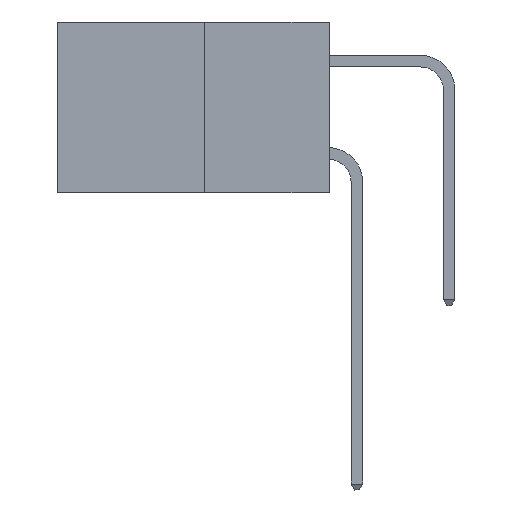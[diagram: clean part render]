
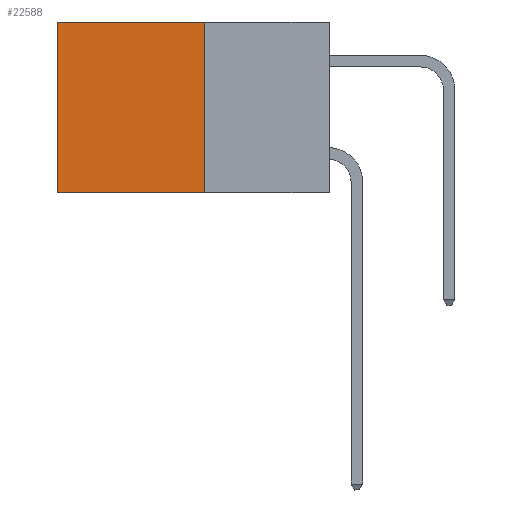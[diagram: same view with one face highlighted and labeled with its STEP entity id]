
A CAD part, left-side view. The second image highlights one B-rep face of the part: STEP entity #22588.
In plain terms, the highlighted planar face has unit normal (-1, 0, 0).
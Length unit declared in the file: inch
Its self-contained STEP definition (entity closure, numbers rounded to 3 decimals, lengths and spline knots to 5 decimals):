
#308 = CARTESIAN_POINT ( 'NONE',  ( 0.277, 0.59, -0.37 ) ) ;
#2342 = LINE ( 'NONE', #20763, #28300 ) ;
#3010 = EDGE_CURVE ( 'NONE', #12105, #6111, #3802, .T. ) ;
#3478 = VECTOR ( 'NONE', #12565, 39.37008 ) ;
#3586 = EDGE_CURVE ( 'NONE', #12547, #6111, #19298, .T. ) ;
#3802 = LINE ( 'NONE', #15116, #10054 ) ;
#4331 = ORIENTED_EDGE ( 'NONE', *, *, #3586, .T. ) ;
#5370 = CARTESIAN_POINT ( 'NONE',  ( 0.277, 0.59, -0.37 ) ) ;
#6111 = VERTEX_POINT ( 'NONE', #5370 ) ;
#6252 = ORIENTED_EDGE ( 'NONE', *, *, #20734, .T. ) ;
#8834 = ORIENTED_EDGE ( 'NONE', *, *, #14954, .F. ) ;
#9442 = DIRECTION ( 'NONE',  ( 1., 0., 0. ) ) ;
#9669 = CARTESIAN_POINT ( 'NONE',  ( 0.277, 0.27, -0.37 ) ) ;
#9868 = CARTESIAN_POINT ( 'NONE',  ( 0.277, 0.27, -0.37 ) ) ;
#10054 = VECTOR ( 'NONE', #14972, 39.37008 ) ;
#11370 = LINE ( 'NONE', #9868, #3478 ) ;
#11796 = FACE_OUTER_BOUND ( 'NONE', #18900, .T. ) ;
#12105 = VERTEX_POINT ( 'NONE', #9669 ) ;
#12182 = AXIS2_PLACEMENT_3D ( 'NONE', #24918, #9442, #27447 ) ;
#12547 = VERTEX_POINT ( 'NONE', #26880 ) ;
#12565 = DIRECTION ( 'NONE',  ( 0., 0., -1. ) ) ;
#12875 = VERTEX_POINT ( 'NONE', #15326 ) ;
#14954 = EDGE_CURVE ( 'NONE', #12875, #12105, #11370, .T. ) ;
#14972 = DIRECTION ( 'NONE',  ( 0., 1., 0. ) ) ;
#15116 = CARTESIAN_POINT ( 'NONE',  ( 0.277, 0.27, -0.37 ) ) ;
#15326 = CARTESIAN_POINT ( 'NONE',  ( 0.277, 0.27, 0. ) ) ;
#17635 = ORIENTED_EDGE ( 'NONE', *, *, #3010, .F. ) ;
#18900 = EDGE_LOOP ( 'NONE', ( #4331, #17635, #8834, #6252 ) ) ;
#19298 = LINE ( 'NONE', #308, #31243 ) ;
#19763 = PLANE ( 'NONE',  #12182 ) ;
#20734 = EDGE_CURVE ( 'NONE', #12875, #12547, #2342, .T. ) ;
#20763 = CARTESIAN_POINT ( 'NONE',  ( 0.277, 0.27, 0. ) ) ;
#22588 = ADVANCED_FACE ( 'NONE', ( #11796 ), #19763, .F. ) ;
#24918 = CARTESIAN_POINT ( 'NONE',  ( 0.277, 0.27, -0.37 ) ) ;
#26880 = CARTESIAN_POINT ( 'NONE',  ( 0.277, 0.59, 0. ) ) ;
#27447 = DIRECTION ( 'NONE',  ( 0., 0., -1. ) ) ;
#28300 = VECTOR ( 'NONE', #33400, 39.37008 ) ;
#30843 = DIRECTION ( 'NONE',  ( 0., 0., -1. ) ) ;
#31243 = VECTOR ( 'NONE', #30843, 39.37008 ) ;
#33400 = DIRECTION ( 'NONE',  ( 0., 1., 0. ) ) ;
